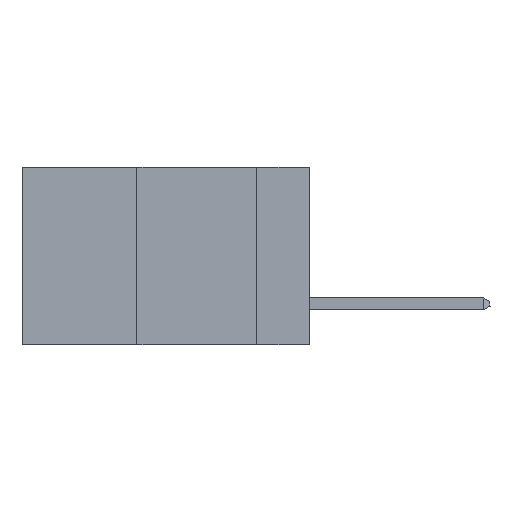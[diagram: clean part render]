
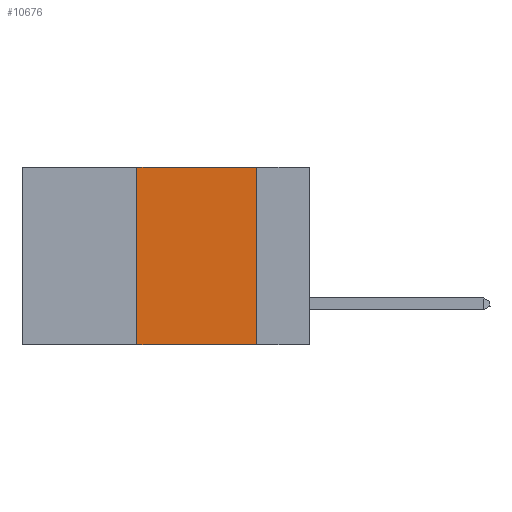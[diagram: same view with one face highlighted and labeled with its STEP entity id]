
A CAD part, left-side view. The second image highlights one B-rep face of the part: STEP entity #10676.
In plain terms, the highlighted planar face has unit normal (-1, 0, 0).
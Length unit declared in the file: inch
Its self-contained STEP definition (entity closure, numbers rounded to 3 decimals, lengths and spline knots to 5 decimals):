
#82 = ORIENTED_EDGE ( 'NONE', *, *, #2023, .F. ) ;
#1436 = ORIENTED_EDGE ( 'NONE', *, *, #10206, .T. ) ;
#1669 = EDGE_LOOP ( 'NONE', ( #9604, #3983, #82, #1436 ) ) ;
#1953 = VERTEX_POINT ( 'NONE', #6782 ) ;
#2023 = EDGE_CURVE ( 'NONE', #1953, #8333, #5371, .T. ) ;
#2111 = VECTOR ( 'NONE', #8612, 39.37008 ) ;
#2120 = CARTESIAN_POINT ( 'NONE',  ( 0., 0.6, -0.37 ) ) ;
#2529 = DIRECTION ( 'NONE',  ( 1., 0., 0. ) ) ;
#2745 = LINE ( 'NONE', #2120, #4947 ) ;
#2761 = CARTESIAN_POINT ( 'NONE',  ( 0., 0.36, 0. ) ) ;
#3633 = VERTEX_POINT ( 'NONE', #5230 ) ;
#3983 = ORIENTED_EDGE ( 'NONE', *, *, #6048, .F. ) ;
#4255 = LINE ( 'NONE', #5907, #7523 ) ;
#4505 = CARTESIAN_POINT ( 'NONE',  ( 0., 0.6, 0. ) ) ;
#4947 = VECTOR ( 'NONE', #8838, 39.37008 ) ;
#5117 = PLANE ( 'NONE',  #8703 ) ;
#5230 = CARTESIAN_POINT ( 'NONE',  ( 0., 0.11, 0. ) ) ;
#5371 = LINE ( 'NONE', #2761, #2111 ) ;
#5586 = CARTESIAN_POINT ( 'NONE',  ( 0., 0.36, 0. ) ) ;
#5591 = VERTEX_POINT ( 'NONE', #6360 ) ;
#5907 = CARTESIAN_POINT ( 'NONE',  ( 0., 0.11, 0. ) ) ;
#6048 = EDGE_CURVE ( 'NONE', #8333, #3633, #9620, .T. ) ;
#6238 = FACE_OUTER_BOUND ( 'NONE', #1669, .T. ) ;
#6360 = CARTESIAN_POINT ( 'NONE',  ( 0., 0.11, -0.37 ) ) ;
#6782 = CARTESIAN_POINT ( 'NONE',  ( 0., 0.36, -0.37 ) ) ;
#6805 = DIRECTION ( 'NONE',  ( 0., 0., -1. ) ) ;
#7002 = EDGE_CURVE ( 'NONE', #3633, #5591, #4255, .T. ) ;
#7426 = VECTOR ( 'NONE', #10326, 39.37008 ) ;
#7523 = VECTOR ( 'NONE', #10092, 39.37008 ) ;
#8333 = VERTEX_POINT ( 'NONE', #5586 ) ;
#8612 = DIRECTION ( 'NONE',  ( 0., 0., 1. ) ) ;
#8703 = AXIS2_PLACEMENT_3D ( 'NONE', #10061, #2529, #6805 ) ;
#8838 = DIRECTION ( 'NONE',  ( 0., -1., 0. ) ) ;
#9604 = ORIENTED_EDGE ( 'NONE', *, *, #7002, .F. ) ;
#9620 = LINE ( 'NONE', #4505, #7426 ) ;
#10061 = CARTESIAN_POINT ( 'NONE',  ( 0., 0.6, 0. ) ) ;
#10092 = DIRECTION ( 'NONE',  ( 0., 0., -1. ) ) ;
#10206 = EDGE_CURVE ( 'NONE', #1953, #5591, #2745, .T. ) ;
#10326 = DIRECTION ( 'NONE',  ( 0., -1., 0. ) ) ;
#10676 = ADVANCED_FACE ( 'NONE', ( #6238 ), #5117, .F. ) ;
